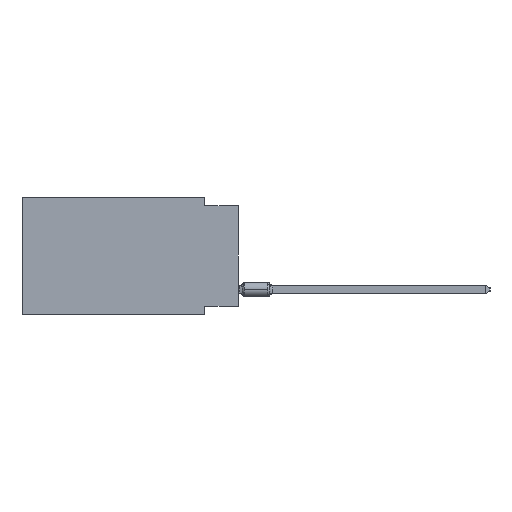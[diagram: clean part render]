
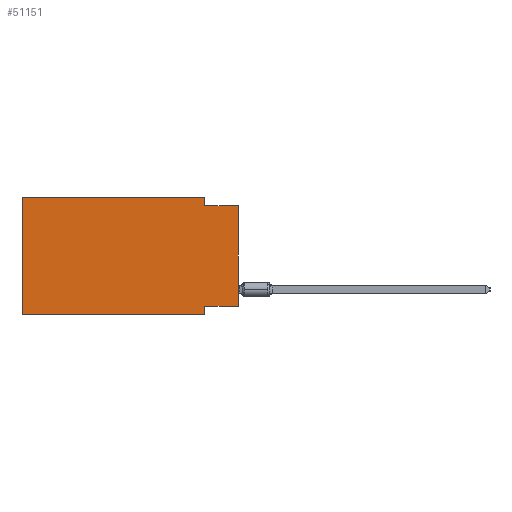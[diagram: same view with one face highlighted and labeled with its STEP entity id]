
A CAD part, left-side view. The second image highlights one B-rep face of the part: STEP entity #51151.
In plain terms, the highlighted planar face has unit normal (-1, 0, 0).
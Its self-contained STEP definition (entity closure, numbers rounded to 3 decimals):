
#36 = CARTESIAN_POINT ( 'NONE',  ( 0., 2.54, -8.89 ) ) ;
#883 = CARTESIAN_POINT ( 'NONE',  ( 0., 16.383, 0. ) ) ;
#1290 = ORIENTED_EDGE ( 'NONE', *, *, #49194, .T. ) ;
#1566 = LINE ( 'NONE', #883, #16938 ) ;
#5169 = ORIENTED_EDGE ( 'NONE', *, *, #68352, .F. ) ;
#7535 = LINE ( 'NONE', #34534, #15851 ) ;
#7931 = ORIENTED_EDGE ( 'NONE', *, *, #13715, .F. ) ;
#10379 = DIRECTION ( 'NONE',  ( 0., -1., 0. ) ) ;
#11030 = VERTEX_POINT ( 'NONE', #20723 ) ;
#11907 = ORIENTED_EDGE ( 'NONE', *, *, #67770, .T. ) ;
#11913 = DIRECTION ( 'NONE',  ( 0., 0., -1. ) ) ;
#12642 = VERTEX_POINT ( 'NONE', #25552 ) ;
#12703 = CARTESIAN_POINT ( 'NONE',  ( 0., 2.54, 0. ) ) ;
#13004 = CARTESIAN_POINT ( 'NONE',  ( 0., 16.383, 0. ) ) ;
#13488 = LINE ( 'NONE', #23319, #44002 ) ;
#13715 = EDGE_CURVE ( 'NONE', #22228, #11030, #23225, .T. ) ;
#15795 = VERTEX_POINT ( 'NONE', #36535 ) ;
#15851 = VECTOR ( 'NONE', #55589, 1000. ) ;
#16938 = VECTOR ( 'NONE', #33465, 1000. ) ;
#17221 = DIRECTION ( 'NONE',  ( 1., 0., 0. ) ) ;
#17382 = CARTESIAN_POINT ( 'NONE',  ( 0., 16.383, 0. ) ) ;
#17816 = EDGE_CURVE ( 'NONE', #45396, #59786, #1566, .T. ) ;
#19021 = VECTOR ( 'NONE', #10379, 1000. ) ;
#19964 = DIRECTION ( 'NONE',  ( 0., 0., -1. ) ) ;
#20723 = CARTESIAN_POINT ( 'NONE',  ( 0., 2.54, -0.635 ) ) ;
#21599 = CARTESIAN_POINT ( 'NONE',  ( 0., 2.54, 0. ) ) ;
#22228 = VERTEX_POINT ( 'NONE', #21599 ) ;
#23225 = LINE ( 'NONE', #12703, #56850 ) ;
#23319 = CARTESIAN_POINT ( 'NONE',  ( 0., 0., 0. ) ) ;
#25552 = CARTESIAN_POINT ( 'NONE',  ( 0., 0., -0.635 ) ) ;
#30292 = LINE ( 'NONE', #51715, #49418 ) ;
#30330 = EDGE_CURVE ( 'NONE', #59786, #22228, #32119, .T. ) ;
#31415 = CARTESIAN_POINT ( 'NONE',  ( 0., 16.383, 0. ) ) ;
#31666 = EDGE_CURVE ( 'NONE', #11030, #12642, #7535, .T. ) ;
#32119 = LINE ( 'NONE', #31415, #19021 ) ;
#33465 = DIRECTION ( 'NONE',  ( 0., 0., 1. ) ) ;
#34534 = CARTESIAN_POINT ( 'NONE',  ( 0., 0., -0.635 ) ) ;
#34593 = ORIENTED_EDGE ( 'NONE', *, *, #17816, .F. ) ;
#35660 = VERTEX_POINT ( 'NONE', #35934 ) ;
#35934 = CARTESIAN_POINT ( 'NONE',  ( 0., 2.54, -8.89 ) ) ;
#36535 = CARTESIAN_POINT ( 'NONE',  ( 0., 2.54, -8.255 ) ) ;
#40289 = CARTESIAN_POINT ( 'NONE',  ( 0., 0., -8.255 ) ) ;
#41185 = DIRECTION ( 'NONE',  ( 0., 1., 0. ) ) ;
#41926 = CARTESIAN_POINT ( 'NONE',  ( 0., 16.383, -8.89 ) ) ;
#43554 = VERTEX_POINT ( 'NONE', #40289 ) ;
#44002 = VECTOR ( 'NONE', #60526, 1000. ) ;
#44189 = LINE ( 'NONE', #36, #60810 ) ;
#45396 = VERTEX_POINT ( 'NONE', #61583 ) ;
#46101 = EDGE_LOOP ( 'NONE', ( #11907, #56428, #7931, #67819, #34593, #1290, #5169, #60260 ) ) ;
#47186 = DIRECTION ( 'NONE',  ( 0., -1., 0. ) ) ;
#49194 = EDGE_CURVE ( 'NONE', #45396, #35660, #67869, .T. ) ;
#49418 = VECTOR ( 'NONE', #41185, 1000. ) ;
#50553 = FACE_OUTER_BOUND ( 'NONE', #46101, .T. ) ;
#51151 = ADVANCED_FACE ( 'NONE', ( #50553 ), #65289, .F. ) ;
#51715 = CARTESIAN_POINT ( 'NONE',  ( 0., 0., -8.255 ) ) ;
#55589 = DIRECTION ( 'NONE',  ( 0., -1., 0. ) ) ;
#56428 = ORIENTED_EDGE ( 'NONE', *, *, #31666, .F. ) ;
#56850 = VECTOR ( 'NONE', #19964, 1000. ) ;
#56956 = AXIS2_PLACEMENT_3D ( 'NONE', #13004, #17221, #65971 ) ;
#59786 = VERTEX_POINT ( 'NONE', #17382 ) ;
#60260 = ORIENTED_EDGE ( 'NONE', *, *, #66590, .F. ) ;
#60526 = DIRECTION ( 'NONE',  ( 0., 0., 1. ) ) ;
#60810 = VECTOR ( 'NONE', #11913, 1000. ) ;
#61583 = CARTESIAN_POINT ( 'NONE',  ( 0., 16.383, -8.89 ) ) ;
#65289 = PLANE ( 'NONE',  #56956 ) ;
#65712 = VECTOR ( 'NONE', #47186, 1000. ) ;
#65971 = DIRECTION ( 'NONE',  ( 0., 0., -1. ) ) ;
#66590 = EDGE_CURVE ( 'NONE', #43554, #15795, #30292, .T. ) ;
#67770 = EDGE_CURVE ( 'NONE', #43554, #12642, #13488, .T. ) ;
#67819 = ORIENTED_EDGE ( 'NONE', *, *, #30330, .F. ) ;
#67869 = LINE ( 'NONE', #41926, #65712 ) ;
#68352 = EDGE_CURVE ( 'NONE', #15795, #35660, #44189, .T. ) ;
